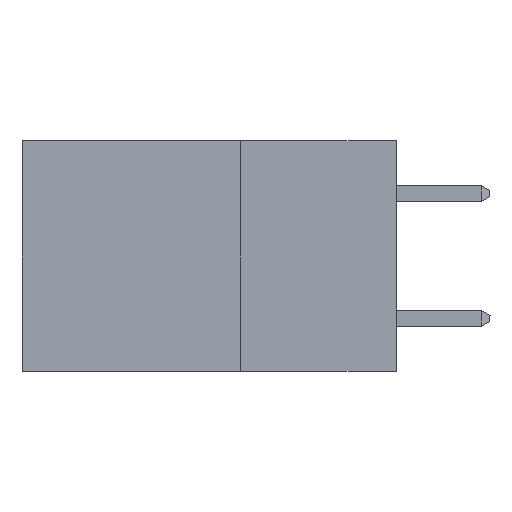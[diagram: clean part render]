
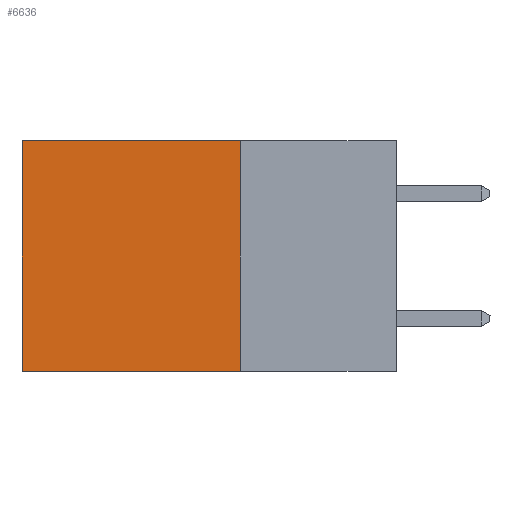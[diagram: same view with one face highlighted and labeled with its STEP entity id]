
A CAD part, left-side view. The second image highlights one B-rep face of the part: STEP entity #6636.
In plain terms, the highlighted planar face has unit normal (-1, 0, 0).
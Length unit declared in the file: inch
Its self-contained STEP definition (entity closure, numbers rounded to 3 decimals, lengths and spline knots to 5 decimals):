
#503 = VECTOR ( 'NONE', #4646, 39.37008 ) ;
#1181 = CARTESIAN_POINT ( 'NONE',  ( 0.2615, 0.25, -0.37 ) ) ;
#1653 = ORIENTED_EDGE ( 'NONE', *, *, #3392, .T. ) ;
#1957 = LINE ( 'NONE', #7518, #9433 ) ;
#2764 = CARTESIAN_POINT ( 'NONE',  ( 0.2615, 0.25, 0. ) ) ;
#2773 = FACE_OUTER_BOUND ( 'NONE', #10370, .T. ) ;
#2947 = EDGE_CURVE ( 'NONE', #11414, #13777, #10426, .T. ) ;
#3392 = EDGE_CURVE ( 'NONE', #14555, #11414, #6146, .T. ) ;
#4016 = CARTESIAN_POINT ( 'NONE',  ( 0.2615, 0.6, -0.37 ) ) ;
#4646 = DIRECTION ( 'NONE',  ( 0., 0., -1. ) ) ;
#4927 = EDGE_CURVE ( 'NONE', #14555, #14865, #11401, .T. ) ;
#5412 = DIRECTION ( 'NONE',  ( 0., 0., -1. ) ) ;
#5431 = VECTOR ( 'NONE', #9689, 39.37008 ) ;
#5455 = DIRECTION ( 'NONE',  ( 1., 0., 0. ) ) ;
#5464 = CARTESIAN_POINT ( 'NONE',  ( 0.2615, 0.25, -0.37 ) ) ;
#5503 = PLANE ( 'NONE',  #6556 ) ;
#6146 = LINE ( 'NONE', #10438, #5431 ) ;
#6556 = AXIS2_PLACEMENT_3D ( 'NONE', #5464, #5455, #5412 ) ;
#6636 = ADVANCED_FACE ( 'NONE', ( #2773 ), #5503, .F. ) ;
#7518 = CARTESIAN_POINT ( 'NONE',  ( 0.2615, 0.25, -0.37 ) ) ;
#7590 = DIRECTION ( 'NONE',  ( 0., 0., -1. ) ) ;
#7699 = CARTESIAN_POINT ( 'NONE',  ( 0.2615, 0.25, -0.37 ) ) ;
#7733 = ORIENTED_EDGE ( 'NONE', *, *, #4927, .F. ) ;
#7755 = DIRECTION ( 'NONE',  ( 0., 1., 0. ) ) ;
#8804 = CARTESIAN_POINT ( 'NONE',  ( 0.2615, 0.6, -0.37 ) ) ;
#9311 = CARTESIAN_POINT ( 'NONE',  ( 0.2615, 0.6, 0. ) ) ;
#9433 = VECTOR ( 'NONE', #7755, 39.37008 ) ;
#9689 = DIRECTION ( 'NONE',  ( 0., 1., 0. ) ) ;
#10370 = EDGE_LOOP ( 'NONE', ( #10407, #13485, #7733, #1653 ) ) ;
#10407 = ORIENTED_EDGE ( 'NONE', *, *, #2947, .T. ) ;
#10426 = LINE ( 'NONE', #4016, #503 ) ;
#10438 = CARTESIAN_POINT ( 'NONE',  ( 0.2615, 0.25, 0. ) ) ;
#11401 = LINE ( 'NONE', #7699, #14117 ) ;
#11414 = VERTEX_POINT ( 'NONE', #9311 ) ;
#13485 = ORIENTED_EDGE ( 'NONE', *, *, #13855, .F. ) ;
#13777 = VERTEX_POINT ( 'NONE', #8804 ) ;
#13855 = EDGE_CURVE ( 'NONE', #14865, #13777, #1957, .T. ) ;
#14117 = VECTOR ( 'NONE', #7590, 39.37008 ) ;
#14555 = VERTEX_POINT ( 'NONE', #2764 ) ;
#14865 = VERTEX_POINT ( 'NONE', #1181 ) ;
